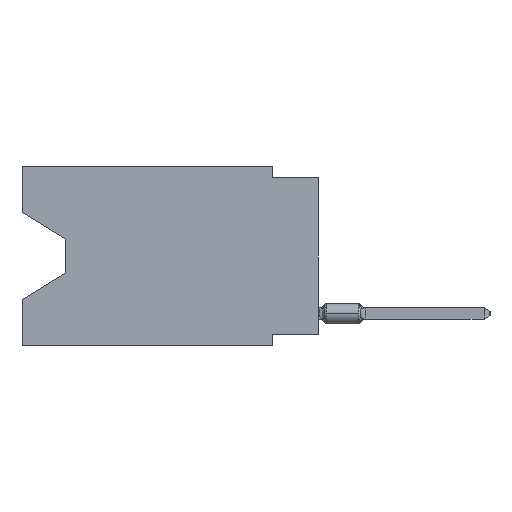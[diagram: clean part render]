
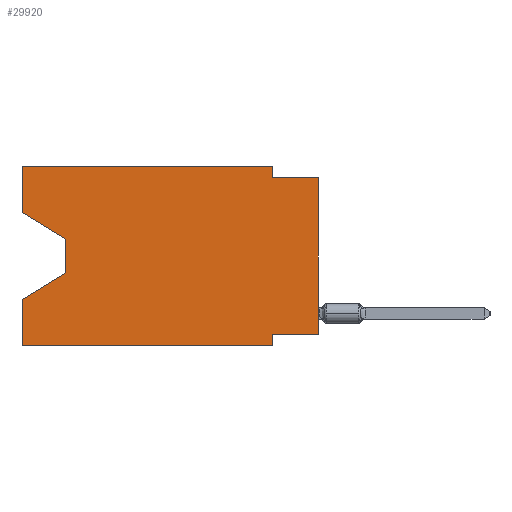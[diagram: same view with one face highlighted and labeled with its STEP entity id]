
A CAD part, left-side view. The second image highlights one B-rep face of the part: STEP entity #29920.
In plain terms, the highlighted planar face has unit normal (-1, 0, 0).
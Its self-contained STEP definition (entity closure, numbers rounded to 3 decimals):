
#1156 = CARTESIAN_POINT ( 'NONE',  ( 0., 16.383, -7.36 ) ) ;
#2112 = ORIENTED_EDGE ( 'NONE', *, *, #57382, .T. ) ;
#2526 = CARTESIAN_POINT ( 'NONE',  ( 0., 2.54, 0. ) ) ;
#4821 = VERTEX_POINT ( 'NONE', #8541 ) ;
#4883 = DIRECTION ( 'NONE',  ( 0., 0., -1. ) ) ;
#6264 = LINE ( 'NONE', #32592, #48732 ) ;
#6979 = CARTESIAN_POINT ( 'NONE',  ( 0., 0., -9.271 ) ) ;
#7586 = ORIENTED_EDGE ( 'NONE', *, *, #19940, .T. ) ;
#7759 = VERTEX_POINT ( 'NONE', #51605 ) ;
#8138 = AXIS2_PLACEMENT_3D ( 'NONE', #64973, #33316, #4883 ) ;
#8265 = ORIENTED_EDGE ( 'NONE', *, *, #31059, .F. ) ;
#8341 = CARTESIAN_POINT ( 'NONE',  ( 0., 0., -9.271 ) ) ;
#8541 = CARTESIAN_POINT ( 'NONE',  ( 0., 16.383, 0. ) ) ;
#9253 = VECTOR ( 'NONE', #30740, 1000. ) ;
#10217 = LINE ( 'NONE', #21602, #10539 ) ;
#10539 = VECTOR ( 'NONE', #26237, 1000. ) ;
#12693 = VECTOR ( 'NONE', #63142, 1000. ) ;
#13460 = VERTEX_POINT ( 'NONE', #1156 ) ;
#14016 = CARTESIAN_POINT ( 'NONE',  ( 0., 16.383, -9.906 ) ) ;
#15667 = EDGE_LOOP ( 'NONE', ( #7586, #55866, #15999, #59185, #18464, #42355, #27662, #2112, #16818, #8265, #20231, #38081 ) ) ;
#15999 = ORIENTED_EDGE ( 'NONE', *, *, #60003, .T. ) ;
#16019 = VERTEX_POINT ( 'NONE', #51240 ) ;
#16035 = VECTOR ( 'NONE', #17738, 1000. ) ;
#16818 = ORIENTED_EDGE ( 'NONE', *, *, #25781, .F. ) ;
#16950 = FACE_OUTER_BOUND ( 'NONE', #15667, .T. ) ;
#17334 = DIRECTION ( 'NONE',  ( 0., -1., 0. ) ) ;
#17696 = CARTESIAN_POINT ( 'NONE',  ( 0., 16.383, -9.906 ) ) ;
#17738 = DIRECTION ( 'NONE',  ( 0., 0., -1. ) ) ;
#18464 = ORIENTED_EDGE ( 'NONE', *, *, #22241, .T. ) ;
#18545 = CARTESIAN_POINT ( 'NONE',  ( 0., 2.54, -0.635 ) ) ;
#19747 = LINE ( 'NONE', #41424, #12693 ) ;
#19940 = EDGE_CURVE ( 'NONE', #32341, #45036, #38563, .T. ) ;
#19983 = DIRECTION ( 'NONE',  ( 0., 0., -1. ) ) ;
#20231 = ORIENTED_EDGE ( 'NONE', *, *, #28032, .F. ) ;
#20488 = VECTOR ( 'NONE', #19983, 1000. ) ;
#21602 = CARTESIAN_POINT ( 'NONE',  ( 0., 13.97, -5.893 ) ) ;
#21859 = DIRECTION ( 'NONE',  ( 0., -1., 0. ) ) ;
#22241 = EDGE_CURVE ( 'NONE', #53096, #16019, #39367, .T. ) ;
#24358 = LINE ( 'NONE', #67741, #20488 ) ;
#24863 = VERTEX_POINT ( 'NONE', #18545 ) ;
#25781 = EDGE_CURVE ( 'NONE', #24863, #62638, #28696, .T. ) ;
#26237 = DIRECTION ( 'NONE',  ( 0., 0.855, -0.519 ) ) ;
#26584 = PLANE ( 'NONE',  #8138 ) ;
#26847 = LINE ( 'NONE', #65238, #60678 ) ;
#26982 = CARTESIAN_POINT ( 'NONE',  ( 0., 2.54, -9.906 ) ) ;
#27662 = ORIENTED_EDGE ( 'NONE', *, *, #44931, .F. ) ;
#28032 = EDGE_CURVE ( 'NONE', #4821, #48678, #26847, .T. ) ;
#28696 = LINE ( 'NONE', #34383, #46997 ) ;
#29920 = ADVANCED_FACE ( 'NONE', ( #16950 ), #26584, .F. ) ;
#30028 = LINE ( 'NONE', #68066, #50887 ) ;
#30055 = VERTEX_POINT ( 'NONE', #6979 ) ;
#30740 = DIRECTION ( 'NONE',  ( 0., 1., 0. ) ) ;
#31059 = EDGE_CURVE ( 'NONE', #48678, #24863, #6264, .T. ) ;
#31094 = CARTESIAN_POINT ( 'NONE',  ( 0., 13.97, -4.013 ) ) ;
#32341 = VERTEX_POINT ( 'NONE', #33748 ) ;
#32592 = CARTESIAN_POINT ( 'NONE',  ( 0., 2.54, 0. ) ) ;
#33316 = DIRECTION ( 'NONE',  ( 1., 0., 0. ) ) ;
#33748 = CARTESIAN_POINT ( 'NONE',  ( 0., 16.383, -2.546 ) ) ;
#34383 = CARTESIAN_POINT ( 'NONE',  ( 0., 0., -0.635 ) ) ;
#34664 = DIRECTION ( 'NONE',  ( 0., 0., 1. ) ) ;
#35768 = VECTOR ( 'NONE', #17334, 1000. ) ;
#35774 = VECTOR ( 'NONE', #55614, 1000. ) ;
#36875 = DIRECTION ( 'NONE',  ( 0., 0., 1. ) ) ;
#37563 = CARTESIAN_POINT ( 'NONE',  ( 0., 16.383, 0. ) ) ;
#38081 = ORIENTED_EDGE ( 'NONE', *, *, #58066, .F. ) ;
#38563 = LINE ( 'NONE', #49226, #35774 ) ;
#39367 = LINE ( 'NONE', #17696, #35768 ) ;
#40054 = DIRECTION ( 'NONE',  ( 0., -1., 0. ) ) ;
#41397 = EDGE_CURVE ( 'NONE', #45036, #52698, #24358, .T. ) ;
#41424 = CARTESIAN_POINT ( 'NONE',  ( 0., 0., 0. ) ) ;
#42355 = ORIENTED_EDGE ( 'NONE', *, *, #56624, .F. ) ;
#44931 = EDGE_CURVE ( 'NONE', #30055, #7759, #57047, .T. ) ;
#45036 = VERTEX_POINT ( 'NONE', #31094 ) ;
#46997 = VECTOR ( 'NONE', #40054, 1000. ) ;
#48678 = VERTEX_POINT ( 'NONE', #2526 ) ;
#48732 = VECTOR ( 'NONE', #59955, 1000. ) ;
#49226 = CARTESIAN_POINT ( 'NONE',  ( 0., 16.383, -2.546 ) ) ;
#50887 = VECTOR ( 'NONE', #34664, 1000. ) ;
#51238 = VECTOR ( 'NONE', #36875, 1000. ) ;
#51240 = CARTESIAN_POINT ( 'NONE',  ( 0., 2.54, -9.906 ) ) ;
#51605 = CARTESIAN_POINT ( 'NONE',  ( 0., 2.54, -9.271 ) ) ;
#52698 = VERTEX_POINT ( 'NONE', #68513 ) ;
#52974 = EDGE_CURVE ( 'NONE', #53096, #13460, #30028, .T. ) ;
#53096 = VERTEX_POINT ( 'NONE', #14016 ) ;
#53210 = LINE ( 'NONE', #37563, #51238 ) ;
#55614 = DIRECTION ( 'NONE',  ( 0., -0.855, -0.519 ) ) ;
#55866 = ORIENTED_EDGE ( 'NONE', *, *, #41397, .T. ) ;
#56512 = CARTESIAN_POINT ( 'NONE',  ( 0., 0., -0.635 ) ) ;
#56624 = EDGE_CURVE ( 'NONE', #7759, #16019, #70362, .T. ) ;
#57047 = LINE ( 'NONE', #8341, #9253 ) ;
#57382 = EDGE_CURVE ( 'NONE', #30055, #62638, #19747, .T. ) ;
#58066 = EDGE_CURVE ( 'NONE', #32341, #4821, #53210, .T. ) ;
#59185 = ORIENTED_EDGE ( 'NONE', *, *, #52974, .F. ) ;
#59955 = DIRECTION ( 'NONE',  ( 0., 0., -1. ) ) ;
#60003 = EDGE_CURVE ( 'NONE', #52698, #13460, #10217, .T. ) ;
#60678 = VECTOR ( 'NONE', #21859, 1000. ) ;
#62638 = VERTEX_POINT ( 'NONE', #56512 ) ;
#63142 = DIRECTION ( 'NONE',  ( 0., 0., 1. ) ) ;
#64973 = CARTESIAN_POINT ( 'NONE',  ( 0., 16.383, 0. ) ) ;
#65238 = CARTESIAN_POINT ( 'NONE',  ( 0., 16.383, 0. ) ) ;
#67741 = CARTESIAN_POINT ( 'NONE',  ( 0., 13.97, -4.013 ) ) ;
#68066 = CARTESIAN_POINT ( 'NONE',  ( 0., 16.383, 0. ) ) ;
#68513 = CARTESIAN_POINT ( 'NONE',  ( 0., 13.97, -5.893 ) ) ;
#70362 = LINE ( 'NONE', #26982, #16035 ) ;
